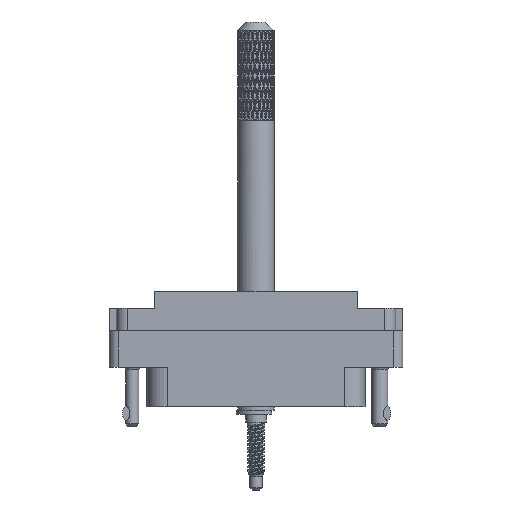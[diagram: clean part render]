
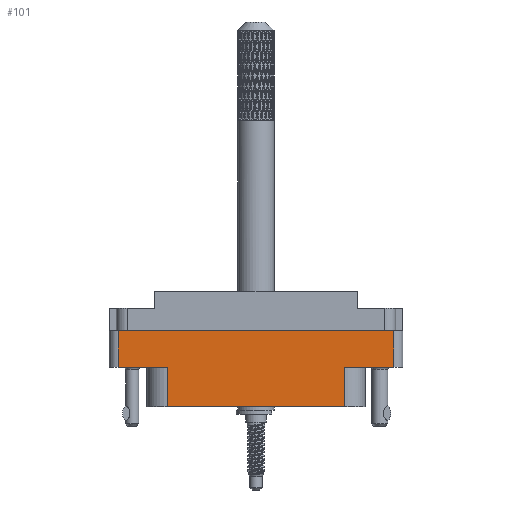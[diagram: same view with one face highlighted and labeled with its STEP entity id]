
A CAD part, front view. The second image highlights one B-rep face of the part: STEP entity #101.
In plain terms, the highlighted planar face has unit normal (0, -1, 0).
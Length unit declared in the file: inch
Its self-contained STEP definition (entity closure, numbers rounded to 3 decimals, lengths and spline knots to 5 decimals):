
#101 = ADVANCED_FACE ( 'NONE', ( #60824 ), #31977, .T. ) ;
#2728 = ORIENTED_EDGE ( 'NONE', *, *, #10912, .T. ) ;
#4027 = ORIENTED_EDGE ( 'NONE', *, *, #68883, .T. ) ;
#6642 = EDGE_CURVE ( 'NONE', #100218, #17390, #69121, .T. ) ;
#10368 = CARTESIAN_POINT ( 'NONE',  ( 0., -0.438, -0.268 ) ) ;
#10487 = DIRECTION ( 'NONE',  ( 0., 0., -1. ) ) ;
#10912 = EDGE_CURVE ( 'NONE', #101654, #58123, #47581, .T. ) ;
#12102 = CARTESIAN_POINT ( 'NONE',  ( 0.938, -0.438, -0.52 ) ) ;
#12518 = LINE ( 'NONE', #45537, #78070 ) ;
#13377 = CARTESIAN_POINT ( 'NONE',  ( 0.938, -0.438, -0.789 ) ) ;
#14078 = CARTESIAN_POINT ( 'NONE',  ( -1., -0.438, -0.789 ) ) ;
#16649 = CARTESIAN_POINT ( 'NONE',  ( 0., -0.438, -0.52 ) ) ;
#17390 = VERTEX_POINT ( 'NONE', #82372 ) ;
#24578 = CARTESIAN_POINT ( 'NONE',  ( -0.938, -0.438, -0.268 ) ) ;
#26604 = CARTESIAN_POINT ( 'NONE',  ( 0.604, -0.438, -0.52 ) ) ;
#28755 = CARTESIAN_POINT ( 'NONE',  ( -0.604, -0.438, -0.789 ) ) ;
#28995 = ORIENTED_EDGE ( 'NONE', *, *, #84853, .F. ) ;
#31977 = PLANE ( 'NONE',  #89893 ) ;
#35284 = ORIENTED_EDGE ( 'NONE', *, *, #74643, .T. ) ;
#37565 = LINE ( 'NONE', #13377, #44053 ) ;
#39577 = EDGE_CURVE ( 'NONE', #100218, #44373, #65784, .T. ) ;
#40784 = VECTOR ( 'NONE', #87689, 39.37008 ) ;
#42374 = CARTESIAN_POINT ( 'NONE',  ( 0.604, -0.438, -0.789 ) ) ;
#42393 = LINE ( 'NONE', #92786, #86972 ) ;
#42573 = DIRECTION ( 'NONE',  ( -1., 0., 0. ) ) ;
#44053 = VECTOR ( 'NONE', #98368, 39.37008 ) ;
#44373 = VERTEX_POINT ( 'NONE', #51709 ) ;
#45537 = CARTESIAN_POINT ( 'NONE',  ( -0.604, -0.438, -0.789 ) ) ;
#47581 = LINE ( 'NONE', #65264, #67355 ) ;
#50165 = VERTEX_POINT ( 'NONE', #66398 ) ;
#51623 = VECTOR ( 'NONE', #42573, 39.37008 ) ;
#51709 = CARTESIAN_POINT ( 'NONE',  ( -0.938, -0.438, -0.52 ) ) ;
#57806 = ORIENTED_EDGE ( 'NONE', *, *, #57971, .T. ) ;
#57971 = EDGE_CURVE ( 'NONE', #106240, #101654, #12518, .T. ) ;
#58123 = VERTEX_POINT ( 'NONE', #42374 ) ;
#60543 = VECTOR ( 'NONE', #10487, 39.37008 ) ;
#60782 = CARTESIAN_POINT ( 'NONE',  ( -0.938, -0.438, -0.789 ) ) ;
#60824 = FACE_OUTER_BOUND ( 'NONE', #62482, .T. ) ;
#62107 = VERTEX_POINT ( 'NONE', #12102 ) ;
#62482 = EDGE_LOOP ( 'NONE', ( #64732, #92183, #82090, #57806, #2728, #4027, #28995, #35284 ) ) ;
#63114 = LINE ( 'NONE', #26604, #40784 ) ;
#64628 = DIRECTION ( 'NONE',  ( 0., 0., -1. ) ) ;
#64732 = ORIENTED_EDGE ( 'NONE', *, *, #6642, .F. ) ;
#65264 = CARTESIAN_POINT ( 'NONE',  ( -1., -0.438, -0.789 ) ) ;
#65627 = DIRECTION ( 'NONE',  ( 1., 0., 0. ) ) ;
#65784 = LINE ( 'NONE', #60782, #60543 ) ;
#66398 = CARTESIAN_POINT ( 'NONE',  ( 0.604, -0.438, -0.52 ) ) ;
#67355 = VECTOR ( 'NONE', #65627, 39.37008 ) ;
#68883 = EDGE_CURVE ( 'NONE', #58123, #50165, #63114, .T. ) ;
#69121 = LINE ( 'NONE', #10368, #90112 ) ;
#72720 = DIRECTION ( 'NONE',  ( 0., -1., 0. ) ) ;
#74643 = EDGE_CURVE ( 'NONE', #62107, #17390, #37565, .T. ) ;
#78070 = VECTOR ( 'NONE', #78582, 39.37008 ) ;
#78582 = DIRECTION ( 'NONE',  ( 0., 0., -1. ) ) ;
#82090 = ORIENTED_EDGE ( 'NONE', *, *, #84886, .T. ) ;
#82372 = CARTESIAN_POINT ( 'NONE',  ( 0.938, -0.438, -0.268 ) ) ;
#84784 = DIRECTION ( 'NONE',  ( 1., 0., 0. ) ) ;
#84853 = EDGE_CURVE ( 'NONE', #62107, #50165, #101441, .T. ) ;
#84886 = EDGE_CURVE ( 'NONE', #44373, #106240, #42393, .T. ) ;
#86972 = VECTOR ( 'NONE', #84784, 39.37008 ) ;
#87689 = DIRECTION ( 'NONE',  ( 0., 0., 1. ) ) ;
#89893 = AXIS2_PLACEMENT_3D ( 'NONE', #14078, #72720, #64628 ) ;
#90112 = VECTOR ( 'NONE', #94644, 39.37008 ) ;
#92183 = ORIENTED_EDGE ( 'NONE', *, *, #39577, .T. ) ;
#92786 = CARTESIAN_POINT ( 'NONE',  ( 0., -0.438, -0.52 ) ) ;
#92887 = CARTESIAN_POINT ( 'NONE',  ( -0.604, -0.438, -0.52 ) ) ;
#94644 = DIRECTION ( 'NONE',  ( 1., 0., 0. ) ) ;
#98368 = DIRECTION ( 'NONE',  ( 0., 0., 1. ) ) ;
#100218 = VERTEX_POINT ( 'NONE', #24578 ) ;
#101441 = LINE ( 'NONE', #16649, #51623 ) ;
#101654 = VERTEX_POINT ( 'NONE', #28755 ) ;
#106240 = VERTEX_POINT ( 'NONE', #92887 ) ;
